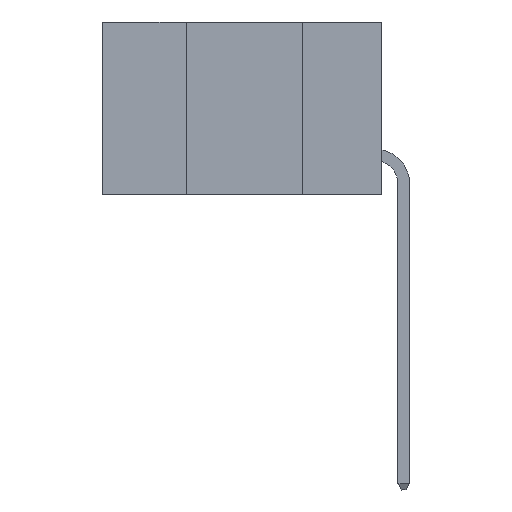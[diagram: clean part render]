
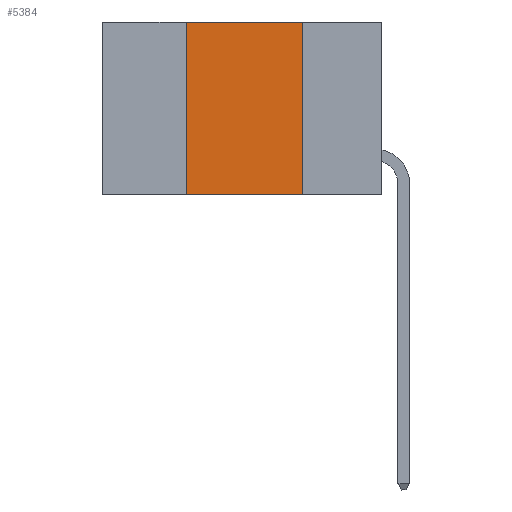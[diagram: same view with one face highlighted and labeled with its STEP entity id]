
A CAD part, left-side view. The second image highlights one B-rep face of the part: STEP entity #5384.
In plain terms, the highlighted planar face has unit normal (-1, 0, 0).
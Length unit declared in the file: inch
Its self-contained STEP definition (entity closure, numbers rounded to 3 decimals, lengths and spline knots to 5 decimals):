
#1214 = CARTESIAN_POINT ( 'NONE',  ( 0., 0.17, -0.37 ) ) ;
#1288 = CARTESIAN_POINT ( 'NONE',  ( 0., 0.17, 0. ) ) ;
#2055 = VERTEX_POINT ( 'NONE', #1288 ) ;
#3325 = EDGE_CURVE ( 'NONE', #8281, #21524, #8875, .T. ) ;
#4980 = LINE ( 'NONE', #9444, #19184 ) ;
#5384 = ADVANCED_FACE ( 'NONE', ( #22733 ), #8250, .F. ) ;
#5803 = LINE ( 'NONE', #18319, #14822 ) ;
#5826 = DIRECTION ( 'NONE',  ( 0., 0., 1. ) ) ;
#6067 = CARTESIAN_POINT ( 'NONE',  ( 0., 0.42, -0.37 ) ) ;
#6106 = VECTOR ( 'NONE', #5826, 39.37008 ) ;
#6154 = VERTEX_POINT ( 'NONE', #22851 ) ;
#7629 = DIRECTION ( 'NONE',  ( 0., 0., -1. ) ) ;
#7651 = DIRECTION ( 'NONE',  ( 1., 0., 0. ) ) ;
#7758 = CARTESIAN_POINT ( 'NONE',  ( 0., 0.6, 0. ) ) ;
#8183 = EDGE_CURVE ( 'NONE', #8281, #6154, #20451, .T. ) ;
#8250 = PLANE ( 'NONE',  #20119 ) ;
#8281 = VERTEX_POINT ( 'NONE', #6067 ) ;
#8300 = VECTOR ( 'NONE', #14204, 39.37008 ) ;
#8875 = LINE ( 'NONE', #14233, #8300 ) ;
#9336 = DIRECTION ( 'NONE',  ( 0., -1., 0. ) ) ;
#9444 = CARTESIAN_POINT ( 'NONE',  ( 0., 0.17, 0. ) ) ;
#12472 = EDGE_CURVE ( 'NONE', #6154, #2055, #5803, .T. ) ;
#14204 = DIRECTION ( 'NONE',  ( 0., -1., 0. ) ) ;
#14233 = CARTESIAN_POINT ( 'NONE',  ( 0., 0.6, -0.37 ) ) ;
#14308 = ORIENTED_EDGE ( 'NONE', *, *, #8183, .F. ) ;
#14822 = VECTOR ( 'NONE', #9336, 39.37008 ) ;
#16445 = ORIENTED_EDGE ( 'NONE', *, *, #22530, .F. ) ;
#16490 = ORIENTED_EDGE ( 'NONE', *, *, #12472, .F. ) ;
#17362 = ORIENTED_EDGE ( 'NONE', *, *, #3325, .T. ) ;
#18319 = CARTESIAN_POINT ( 'NONE',  ( 0., 0.6, 0. ) ) ;
#19184 = VECTOR ( 'NONE', #21921, 39.37008 ) ;
#20119 = AXIS2_PLACEMENT_3D ( 'NONE', #7758, #7651, #7629 ) ;
#20158 = CARTESIAN_POINT ( 'NONE',  ( 0., 0.42, 0. ) ) ;
#20416 = EDGE_LOOP ( 'NONE', ( #16445, #16490, #14308, #17362 ) ) ;
#20451 = LINE ( 'NONE', #20158, #6106 ) ;
#21524 = VERTEX_POINT ( 'NONE', #1214 ) ;
#21921 = DIRECTION ( 'NONE',  ( 0., 0., -1. ) ) ;
#22530 = EDGE_CURVE ( 'NONE', #2055, #21524, #4980, .T. ) ;
#22733 = FACE_OUTER_BOUND ( 'NONE', #20416, .T. ) ;
#22851 = CARTESIAN_POINT ( 'NONE',  ( 0., 0.42, 0. ) ) ;
